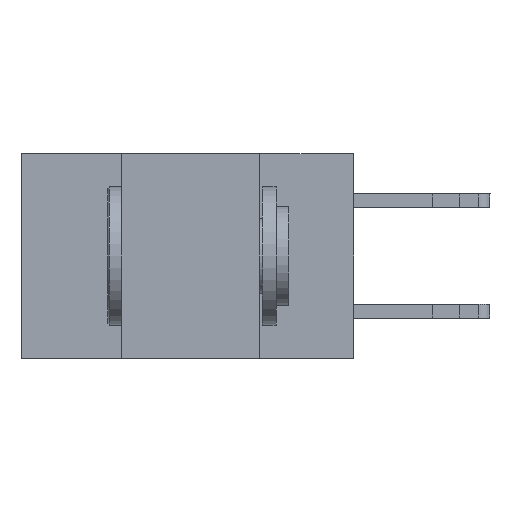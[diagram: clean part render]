
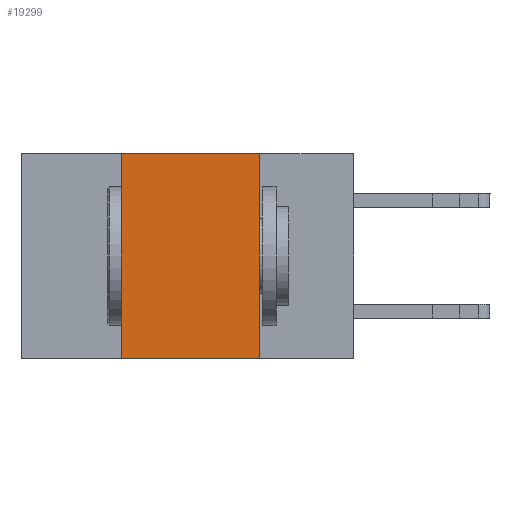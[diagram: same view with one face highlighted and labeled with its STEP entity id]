
A CAD part, left-side view. The second image highlights one B-rep face of the part: STEP entity #19299.
In plain terms, the highlighted planar face has unit normal (-1, 0, 0).
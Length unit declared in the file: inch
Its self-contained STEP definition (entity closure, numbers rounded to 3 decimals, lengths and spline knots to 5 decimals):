
#479 = VECTOR ( 'NONE', #13428, 39.37008 ) ;
#2815 = ORIENTED_EDGE ( 'NONE', *, *, #3164, .F. ) ;
#3164 = EDGE_CURVE ( 'NONE', #25116, #11743, #6665, .T. ) ;
#3620 = ORIENTED_EDGE ( 'NONE', *, *, #22144, .T. ) ;
#3855 = LINE ( 'NONE', #7354, #20444 ) ;
#4536 = LINE ( 'NONE', #15699, #479 ) ;
#6474 = DIRECTION ( 'NONE',  ( 0., -1., 0. ) ) ;
#6665 = LINE ( 'NONE', #18432, #24531 ) ;
#7354 = CARTESIAN_POINT ( 'NONE',  ( 0., 0.42, 0. ) ) ;
#8066 = EDGE_CURVE ( 'NONE', #22619, #25116, #3855, .T. ) ;
#9374 = DIRECTION ( 'NONE',  ( 0., 0., 1. ) ) ;
#9892 = FACE_OUTER_BOUND ( 'NONE', #22674, .T. ) ;
#11743 = VERTEX_POINT ( 'NONE', #23512 ) ;
#12182 = CARTESIAN_POINT ( 'NONE',  ( 0., 0.6, -0.37 ) ) ;
#13428 = DIRECTION ( 'NONE',  ( 0., 0., -1. ) ) ;
#13508 = PLANE ( 'NONE',  #21662 ) ;
#13770 = DIRECTION ( 'NONE',  ( 0., 0., -1. ) ) ;
#14912 = CARTESIAN_POINT ( 'NONE',  ( 0., 0.42, -0.37 ) ) ;
#15042 = VECTOR ( 'NONE', #20163, 39.37008 ) ;
#15699 = CARTESIAN_POINT ( 'NONE',  ( 0., 0.17, 0. ) ) ;
#15777 = DIRECTION ( 'NONE',  ( 1., 0., 0. ) ) ;
#15799 = VERTEX_POINT ( 'NONE', #18741 ) ;
#15934 = ORIENTED_EDGE ( 'NONE', *, *, #8066, .F. ) ;
#18432 = CARTESIAN_POINT ( 'NONE',  ( 0., 0.6, 0. ) ) ;
#18741 = CARTESIAN_POINT ( 'NONE',  ( 0., 0.17, -0.37 ) ) ;
#18982 = CARTESIAN_POINT ( 'NONE',  ( 0., 0.42, 0. ) ) ;
#19299 = ADVANCED_FACE ( 'NONE', ( #9892 ), #13508, .F. ) ;
#20055 = EDGE_CURVE ( 'NONE', #11743, #15799, #4536, .T. ) ;
#20163 = DIRECTION ( 'NONE',  ( 0., -1., 0. ) ) ;
#20376 = LINE ( 'NONE', #12182, #15042 ) ;
#20444 = VECTOR ( 'NONE', #9374, 39.37008 ) ;
#21662 = AXIS2_PLACEMENT_3D ( 'NONE', #25667, #15777, #13770 ) ;
#22144 = EDGE_CURVE ( 'NONE', #22619, #15799, #20376, .T. ) ;
#22619 = VERTEX_POINT ( 'NONE', #14912 ) ;
#22674 = EDGE_LOOP ( 'NONE', ( #22850, #2815, #15934, #3620 ) ) ;
#22850 = ORIENTED_EDGE ( 'NONE', *, *, #20055, .F. ) ;
#23512 = CARTESIAN_POINT ( 'NONE',  ( 0., 0.17, 0. ) ) ;
#24531 = VECTOR ( 'NONE', #6474, 39.37008 ) ;
#25116 = VERTEX_POINT ( 'NONE', #18982 ) ;
#25667 = CARTESIAN_POINT ( 'NONE',  ( 0., 0.6, 0. ) ) ;
